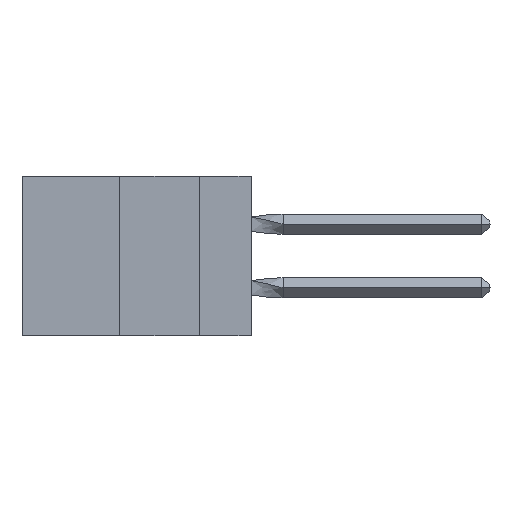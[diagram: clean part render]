
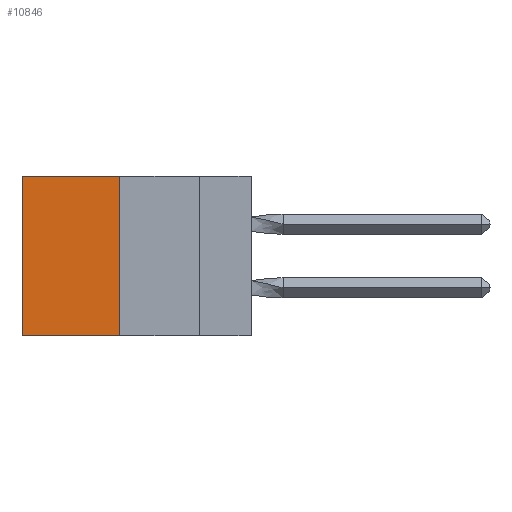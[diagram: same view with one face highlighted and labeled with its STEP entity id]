
A CAD part, left-side view. The second image highlights one B-rep face of the part: STEP entity #10846.
In plain terms, the highlighted planar face has unit normal (-1, 0, 0).
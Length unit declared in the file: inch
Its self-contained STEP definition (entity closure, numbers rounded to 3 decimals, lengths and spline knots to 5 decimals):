
#637 = DIRECTION ( 'NONE',  ( 0., 1., 0. ) ) ;
#1087 = VECTOR ( 'NONE', #11186, 39.37008 ) ;
#1328 = VERTEX_POINT ( 'NONE', #11022 ) ;
#1773 = DIRECTION ( 'NONE',  ( 0., 1., 0. ) ) ;
#1844 = VERTEX_POINT ( 'NONE', #12866 ) ;
#2052 = CARTESIAN_POINT ( 'NONE',  ( 0.305, 0.72, -0.5 ) ) ;
#2288 = DIRECTION ( 'NONE',  ( 1., 0., 0. ) ) ;
#2604 = CARTESIAN_POINT ( 'NONE',  ( 0.305, 0.413, -0.5 ) ) ;
#3138 = CARTESIAN_POINT ( 'NONE',  ( 0.305, 0.413, -0.5 ) ) ;
#3851 = EDGE_CURVE ( 'NONE', #4566, #1328, #4102, .T. ) ;
#4102 = LINE ( 'NONE', #13222, #9478 ) ;
#4162 = LINE ( 'NONE', #2604, #9536 ) ;
#4566 = VERTEX_POINT ( 'NONE', #5620 ) ;
#4690 = LINE ( 'NONE', #2052, #1087 ) ;
#5209 = VERTEX_POINT ( 'NONE', #3138 ) ;
#5620 = CARTESIAN_POINT ( 'NONE',  ( 0.305, 0.413, 0. ) ) ;
#5817 = ORIENTED_EDGE ( 'NONE', *, *, #12408, .T. ) ;
#6262 = AXIS2_PLACEMENT_3D ( 'NONE', #9168, #2288, #10332 ) ;
#7787 = EDGE_LOOP ( 'NONE', ( #5817, #12031, #10482, #11314 ) ) ;
#8285 = VECTOR ( 'NONE', #1773, 39.37008 ) ;
#8414 = DIRECTION ( 'NONE',  ( 0., 0., -1. ) ) ;
#8665 = CARTESIAN_POINT ( 'NONE',  ( 0.305, 0.413, -0.5 ) ) ;
#9168 = CARTESIAN_POINT ( 'NONE',  ( 0.305, 0.413, -0.5 ) ) ;
#9478 = VECTOR ( 'NONE', #637, 39.37008 ) ;
#9536 = VECTOR ( 'NONE', #8414, 39.37008 ) ;
#10332 = DIRECTION ( 'NONE',  ( 0., 0., -1. ) ) ;
#10482 = ORIENTED_EDGE ( 'NONE', *, *, #11242, .F. ) ;
#10846 = ADVANCED_FACE ( 'NONE', ( #10983 ), #12770, .F. ) ;
#10983 = FACE_OUTER_BOUND ( 'NONE', #7787, .T. ) ;
#11022 = CARTESIAN_POINT ( 'NONE',  ( 0.305, 0.72, 0. ) ) ;
#11186 = DIRECTION ( 'NONE',  ( 0., 0., -1. ) ) ;
#11242 = EDGE_CURVE ( 'NONE', #4566, #5209, #4162, .T. ) ;
#11314 = ORIENTED_EDGE ( 'NONE', *, *, #3851, .T. ) ;
#11801 = EDGE_CURVE ( 'NONE', #5209, #1844, #12758, .T. ) ;
#12031 = ORIENTED_EDGE ( 'NONE', *, *, #11801, .F. ) ;
#12408 = EDGE_CURVE ( 'NONE', #1328, #1844, #4690, .T. ) ;
#12758 = LINE ( 'NONE', #8665, #8285 ) ;
#12770 = PLANE ( 'NONE',  #6262 ) ;
#12866 = CARTESIAN_POINT ( 'NONE',  ( 0.305, 0.72, -0.5 ) ) ;
#13222 = CARTESIAN_POINT ( 'NONE',  ( 0.305, 0.413, 0. ) ) ;
